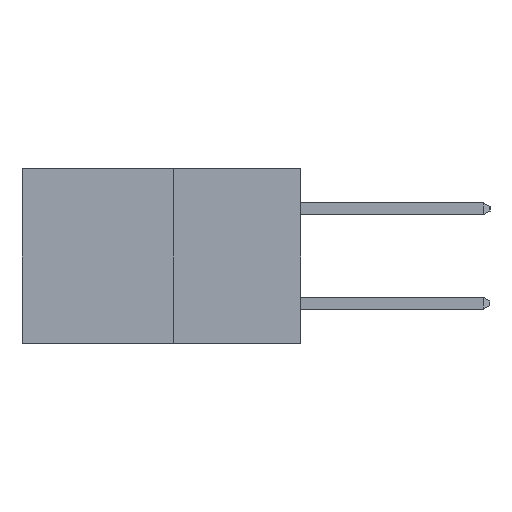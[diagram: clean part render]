
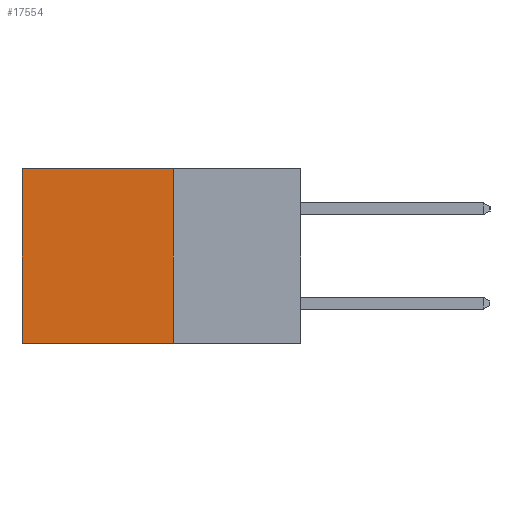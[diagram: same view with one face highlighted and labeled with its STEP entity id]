
A CAD part, left-side view. The second image highlights one B-rep face of the part: STEP entity #17554.
In plain terms, the highlighted planar face has unit normal (-1, 0, 0).
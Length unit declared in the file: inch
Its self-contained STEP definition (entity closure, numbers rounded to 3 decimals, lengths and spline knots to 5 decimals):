
#274 = CARTESIAN_POINT ( 'NONE',  ( 0.277, 0.27, -0.37 ) ) ;
#1041 = VECTOR ( 'NONE', #5239, 39.37008 ) ;
#2259 = EDGE_CURVE ( 'NONE', #16027, #28290, #14055, .T. ) ;
#2698 = EDGE_CURVE ( 'NONE', #28290, #22850, #7550, .T. ) ;
#3423 = DIRECTION ( 'NONE',  ( 1., 0., 0. ) ) ;
#4409 = FACE_OUTER_BOUND ( 'NONE', #13740, .T. ) ;
#5239 = DIRECTION ( 'NONE',  ( 0., 1., 0. ) ) ;
#5391 = ORIENTED_EDGE ( 'NONE', *, *, #14802, .T. ) ;
#5726 = CARTESIAN_POINT ( 'NONE',  ( 0.277, 0.27, 0. ) ) ;
#6292 = CARTESIAN_POINT ( 'NONE',  ( 0.277, 0.59, 0. ) ) ;
#6627 = LINE ( 'NONE', #26175, #18940 ) ;
#7550 = LINE ( 'NONE', #14575, #1041 ) ;
#7565 = CARTESIAN_POINT ( 'NONE',  ( 0.277, 0.27, 0. ) ) ;
#7577 = VECTOR ( 'NONE', #18837, 39.37008 ) ;
#8145 = DIRECTION ( 'NONE',  ( 0., 1., 0. ) ) ;
#11852 = VECTOR ( 'NONE', #8145, 39.37008 ) ;
#12985 = EDGE_CURVE ( 'NONE', #22420, #22850, #6627, .T. ) ;
#13740 = EDGE_LOOP ( 'NONE', ( #15301, #14871, #17630, #5391 ) ) ;
#14055 = LINE ( 'NONE', #19278, #7577 ) ;
#14575 = CARTESIAN_POINT ( 'NONE',  ( 0.277, 0.27, -0.37 ) ) ;
#14802 = EDGE_CURVE ( 'NONE', #16027, #22420, #25043, .T. ) ;
#14871 = ORIENTED_EDGE ( 'NONE', *, *, #2698, .F. ) ;
#15301 = ORIENTED_EDGE ( 'NONE', *, *, #12985, .T. ) ;
#15650 = CARTESIAN_POINT ( 'NONE',  ( 0.277, 0.27, -0.37 ) ) ;
#16027 = VERTEX_POINT ( 'NONE', #7565 ) ;
#17554 = ADVANCED_FACE ( 'NONE', ( #4409 ), #18134, .F. ) ;
#17630 = ORIENTED_EDGE ( 'NONE', *, *, #2259, .F. ) ;
#17761 = CARTESIAN_POINT ( 'NONE',  ( 0.277, 0.59, -0.37 ) ) ;
#18134 = PLANE ( 'NONE',  #19919 ) ;
#18837 = DIRECTION ( 'NONE',  ( 0., 0., -1. ) ) ;
#18940 = VECTOR ( 'NONE', #28578, 39.37008 ) ;
#19278 = CARTESIAN_POINT ( 'NONE',  ( 0.277, 0.27, -0.37 ) ) ;
#19919 = AXIS2_PLACEMENT_3D ( 'NONE', #15650, #3423, #20607 ) ;
#20607 = DIRECTION ( 'NONE',  ( 0., 0., -1. ) ) ;
#22420 = VERTEX_POINT ( 'NONE', #6292 ) ;
#22850 = VERTEX_POINT ( 'NONE', #17761 ) ;
#25043 = LINE ( 'NONE', #5726, #11852 ) ;
#26175 = CARTESIAN_POINT ( 'NONE',  ( 0.277, 0.59, -0.37 ) ) ;
#28290 = VERTEX_POINT ( 'NONE', #274 ) ;
#28578 = DIRECTION ( 'NONE',  ( 0., 0., -1. ) ) ;
